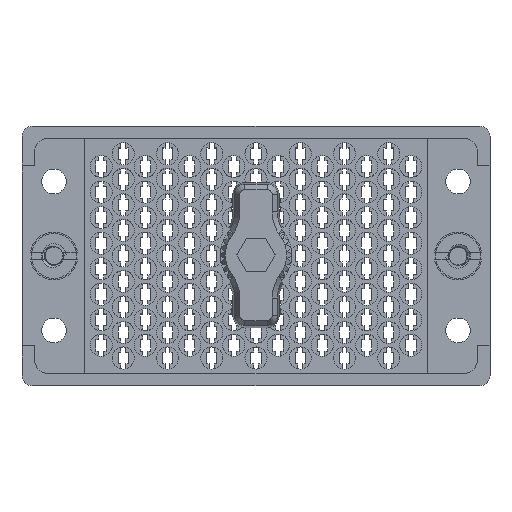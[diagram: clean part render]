
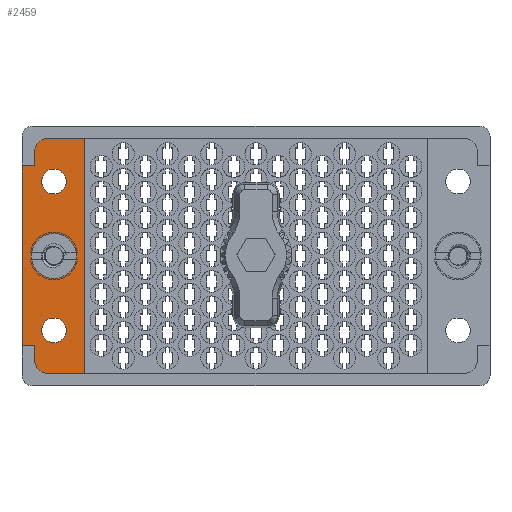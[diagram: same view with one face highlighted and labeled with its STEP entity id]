
A CAD part, top view. The second image highlights one B-rep face of the part: STEP entity #2459.
In plain terms, the highlighted planar face has unit normal (0, 0, 1).
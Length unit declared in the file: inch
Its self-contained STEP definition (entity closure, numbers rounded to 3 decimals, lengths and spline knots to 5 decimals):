
#202 = DIRECTION ( 'NONE',  ( 0., 0., 1. ) ) ;
#1156 = AXIS2_PLACEMENT_3D ( 'NONE', #48241, #108371, #100209 ) ;
#2459 = ADVANCED_FACE ( 'NONE', ( #61265, #38686, #32164, #97308 ), #48688, .T. ) ;
#4063 = DIRECTION ( 'NONE',  ( 0., 0., 1. ) ) ;
#4289 = EDGE_CURVE ( 'NONE', #85625, #64755, #30792, .T. ) ;
#6170 = ORIENTED_EDGE ( 'NONE', *, *, #50398, .F. ) ;
#6669 = CARTESIAN_POINT ( 'NONE',  ( -1.26, 0.4375, -0.117 ) ) ;
#8093 = CIRCLE ( 'NONE', #88939, 0.075 ) ;
#9647 = EDGE_LOOP ( 'NONE', ( #76361, #94280 ) ) ;
#10760 = ORIENTED_EDGE ( 'NONE', *, *, #34440, .T. ) ;
#11566 = LINE ( 'NONE', #105293, #71354 ) ;
#12044 = ORIENTED_EDGE ( 'NONE', *, *, #94939, .T. ) ;
#12897 = CARTESIAN_POINT ( 'NONE',  ( -1.3, 0., -0.117 ) ) ;
#13756 = CARTESIAN_POINT ( 'NONE',  ( -1.225, 0.69, -0.117 ) ) ;
#14881 = DIRECTION ( 'NONE',  ( 1., 0., 0. ) ) ;
#16908 = LINE ( 'NONE', #58837, #104635 ) ;
#18462 = LINE ( 'NONE', #58819, #83582 ) ;
#19349 = DIRECTION ( 'NONE',  ( 0., 0., 1. ) ) ;
#20358 = AXIS2_PLACEMENT_3D ( 'NONE', #100452, #58110, #75189 ) ;
#21151 = DIRECTION ( 'NONE',  ( 1., 0., 0. ) ) ;
#21687 = DIRECTION ( 'NONE',  ( 1., 0., 0. ) ) ;
#23961 = EDGE_LOOP ( 'NONE', ( #100579, #12044, #10760, #46238, #97655, #6170, #43141, #68533, #96807, #47739 ) ) ;
#24908 = CARTESIAN_POINT ( 'NONE',  ( -1.32, 0., -0.117 ) ) ;
#25008 = VERTEX_POINT ( 'NONE', #60267 ) ;
#25371 = VERTEX_POINT ( 'NONE', #107013 ) ;
#26425 = EDGE_LOOP ( 'NONE', ( #42098, #32777 ) ) ;
#26443 = LINE ( 'NONE', #81622, #51700 ) ;
#27898 = CARTESIAN_POINT ( 'NONE',  ( -1.1875, -0.4375, -0.117 ) ) ;
#30718 = EDGE_CURVE ( 'NONE', #97364, #71471, #67010, .T. ) ;
#30792 = LINE ( 'NONE', #44083, #95869 ) ;
#30960 = CARTESIAN_POINT ( 'NONE',  ( -1.005, 0.69, -0.117 ) ) ;
#32164 = FACE_BOUND ( 'NONE', #9647, .T. ) ;
#32777 = ORIENTED_EDGE ( 'NONE', *, *, #61422, .F. ) ;
#33132 = EDGE_CURVE ( 'NONE', #85235, #85625, #18462, .T. ) ;
#33253 = CIRCLE ( 'NONE', #103457, 0.0725 ) ;
#33356 = VECTOR ( 'NONE', #58072, 39.37008 ) ;
#33606 = VERTEX_POINT ( 'NONE', #6669 ) ;
#33649 = VERTEX_POINT ( 'NONE', #67560 ) ;
#33679 = LINE ( 'NONE', #75118, #60197 ) ;
#34440 = EDGE_CURVE ( 'NONE', #106465, #25008, #11566, .T. ) ;
#34630 = LINE ( 'NONE', #100408, #33356 ) ;
#36537 = AXIS2_PLACEMENT_3D ( 'NONE', #27898, #19349, #95850 ) ;
#37973 = DIRECTION ( 'NONE',  ( 1., 0., 0. ) ) ;
#38686 = FACE_BOUND ( 'NONE', #26425, .T. ) ;
#42098 = ORIENTED_EDGE ( 'NONE', *, *, #30718, .F. ) ;
#43141 = ORIENTED_EDGE ( 'NONE', *, *, #59621, .T. ) ;
#44083 = CARTESIAN_POINT ( 'NONE',  ( 0., 0.69, -0.117 ) ) ;
#44820 = DIRECTION ( 'NONE',  ( -1., 0., 0. ) ) ;
#46238 = ORIENTED_EDGE ( 'NONE', *, *, #93476, .T. ) ;
#47739 = ORIENTED_EDGE ( 'NONE', *, *, #33132, .T. ) ;
#47819 = EDGE_LOOP ( 'NONE', ( #90744, #95630 ) ) ;
#48241 = CARTESIAN_POINT ( 'NONE',  ( -1.225, 0.615, -0.117 ) ) ;
#48542 = AXIS2_PLACEMENT_3D ( 'NONE', #62396, #4063, #21151 ) ;
#48688 = PLANE ( 'NONE',  #60248 ) ;
#49027 = EDGE_CURVE ( 'NONE', #33649, #51265, #33679, .T. ) ;
#50398 = EDGE_CURVE ( 'NONE', #25371, #51265, #34630, .T. ) ;
#50629 = DIRECTION ( 'NONE',  ( 0., 1., 0. ) ) ;
#50853 = EDGE_CURVE ( 'NONE', #98989, #72801, #85011, .T. ) ;
#51251 = CARTESIAN_POINT ( 'NONE',  ( -1.3, -0.615, -0.117 ) ) ;
#51265 = VERTEX_POINT ( 'NONE', #78604 ) ;
#51700 = VECTOR ( 'NONE', #73082, 39.37008 ) ;
#53683 = DIRECTION ( 'NONE',  ( 0., -1., 0. ) ) ;
#55628 = DIRECTION ( 'NONE',  ( 0., -1., 0. ) ) ;
#56229 = DIRECTION ( 'NONE',  ( 0., 0., 1. ) ) ;
#58072 = DIRECTION ( 'NONE',  ( -1., 0., 0. ) ) ;
#58110 = DIRECTION ( 'NONE',  ( 0., 0., 1. ) ) ;
#58331 = DIRECTION ( 'NONE',  ( 0., 0., 1. ) ) ;
#58819 = CARTESIAN_POINT ( 'NONE',  ( -1.005, 0.7625, -0.117 ) ) ;
#58837 = CARTESIAN_POINT ( 'NONE',  ( 0., -0.69, -0.117 ) ) ;
#59216 = AXIS2_PLACEMENT_3D ( 'NONE', #93768, #202, #68166 ) ;
#59621 = EDGE_CURVE ( 'NONE', #25371, #102168, #61151, .T. ) ;
#60197 = VECTOR ( 'NONE', #74015, 39.37008 ) ;
#60248 = AXIS2_PLACEMENT_3D ( 'NONE', #108091, #58331, #14881 ) ;
#60267 = CARTESIAN_POINT ( 'NONE',  ( -1.3, 0.5285, -0.117 ) ) ;
#61151 = LINE ( 'NONE', #12897, #66470 ) ;
#61265 = FACE_BOUND ( 'NONE', #47819, .T. ) ;
#61422 = EDGE_CURVE ( 'NONE', #71471, #97364, #64324, .T. ) ;
#62396 = CARTESIAN_POINT ( 'NONE',  ( -1.1875, 0., -0.117 ) ) ;
#64324 = CIRCLE ( 'NONE', #36537, 0.0725 ) ;
#64660 = DIRECTION ( 'NONE',  ( 0., 0., 1. ) ) ;
#64667 = VERTEX_POINT ( 'NONE', #79921 ) ;
#64755 = VERTEX_POINT ( 'NONE', #13756 ) ;
#65998 = CIRCLE ( 'NONE', #1156, 0.075 ) ;
#66470 = VECTOR ( 'NONE', #55628, 39.37008 ) ;
#66790 = DIRECTION ( 'NONE',  ( 1., 0., 0. ) ) ;
#67010 = CIRCLE ( 'NONE', #59216, 0.0725 ) ;
#67349 = DIRECTION ( 'NONE',  ( -1., 0., 0. ) ) ;
#67560 = CARTESIAN_POINT ( 'NONE',  ( -1.375, 0.5285, -0.117 ) ) ;
#68004 = CARTESIAN_POINT ( 'NONE',  ( -1.115, -0.4375, -0.117 ) ) ;
#68166 = DIRECTION ( 'NONE',  ( 1., 0., 0. ) ) ;
#68533 = ORIENTED_EDGE ( 'NONE', *, *, #75363, .T. ) ;
#69321 = CIRCLE ( 'NONE', #20358, 0.1325 ) ;
#69415 = CARTESIAN_POINT ( 'NONE',  ( -1.26, -0.4375, -0.117 ) ) ;
#71354 = VECTOR ( 'NONE', #53683, 39.37008 ) ;
#71471 = VERTEX_POINT ( 'NONE', #68004 ) ;
#72801 = VERTEX_POINT ( 'NONE', #79033 ) ;
#73082 = DIRECTION ( 'NONE',  ( -1., 0., 0. ) ) ;
#73471 = EDGE_CURVE ( 'NONE', #33606, #64667, #93384, .T. ) ;
#74015 = DIRECTION ( 'NONE',  ( 0., -1., 0. ) ) ;
#75118 = CARTESIAN_POINT ( 'NONE',  ( -1.375, 0.7625, -0.117 ) ) ;
#75189 = DIRECTION ( 'NONE',  ( 1., 0., 0. ) ) ;
#75363 = EDGE_CURVE ( 'NONE', #102168, #97219, #8093, .T. ) ;
#76361 = ORIENTED_EDGE ( 'NONE', *, *, #104033, .F. ) ;
#77356 = CARTESIAN_POINT ( 'NONE',  ( -1.3, 0.615, -0.117 ) ) ;
#78604 = CARTESIAN_POINT ( 'NONE',  ( -1.375, -0.5285, -0.117 ) ) ;
#79033 = CARTESIAN_POINT ( 'NONE',  ( -1.055, 0., -0.117 ) ) ;
#79921 = CARTESIAN_POINT ( 'NONE',  ( -1.115, 0.4375, -0.117 ) ) ;
#81622 = CARTESIAN_POINT ( 'NONE',  ( 0., 0.5285, -0.117 ) ) ;
#83582 = VECTOR ( 'NONE', #50629, 39.37008 ) ;
#85011 = CIRCLE ( 'NONE', #48542, 0.1325 ) ;
#85235 = VERTEX_POINT ( 'NONE', #93771 ) ;
#85625 = VERTEX_POINT ( 'NONE', #30960 ) ;
#88939 = AXIS2_PLACEMENT_3D ( 'NONE', #92739, #109125, #66790 ) ;
#90744 = ORIENTED_EDGE ( 'NONE', *, *, #73471, .F. ) ;
#92422 = CARTESIAN_POINT ( 'NONE',  ( -1.225, -0.69, -0.117 ) ) ;
#92444 = AXIS2_PLACEMENT_3D ( 'NONE', #107095, #56229, #21687 ) ;
#92739 = CARTESIAN_POINT ( 'NONE',  ( -1.225, -0.615, -0.117 ) ) ;
#92798 = EDGE_CURVE ( 'NONE', #64667, #33606, #33253, .T. ) ;
#93384 = CIRCLE ( 'NONE', #92444, 0.0725 ) ;
#93476 = EDGE_CURVE ( 'NONE', #25008, #33649, #26443, .T. ) ;
#93768 = CARTESIAN_POINT ( 'NONE',  ( -1.1875, -0.4375, -0.117 ) ) ;
#93771 = CARTESIAN_POINT ( 'NONE',  ( -1.005, -0.69, -0.117 ) ) ;
#94280 = ORIENTED_EDGE ( 'NONE', *, *, #50853, .F. ) ;
#94939 = EDGE_CURVE ( 'NONE', #64755, #106465, #65998, .T. ) ;
#95630 = ORIENTED_EDGE ( 'NONE', *, *, #92798, .F. ) ;
#95850 = DIRECTION ( 'NONE',  ( 1., 0., 0. ) ) ;
#95869 = VECTOR ( 'NONE', #44820, 39.37008 ) ;
#96807 = ORIENTED_EDGE ( 'NONE', *, *, #109407, .F. ) ;
#97219 = VERTEX_POINT ( 'NONE', #92422 ) ;
#97308 = FACE_OUTER_BOUND ( 'NONE', #23961, .T. ) ;
#97364 = VERTEX_POINT ( 'NONE', #69415 ) ;
#97655 = ORIENTED_EDGE ( 'NONE', *, *, #49027, .T. ) ;
#98989 = VERTEX_POINT ( 'NONE', #24908 ) ;
#100209 = DIRECTION ( 'NONE',  ( 1., 0., 0. ) ) ;
#100408 = CARTESIAN_POINT ( 'NONE',  ( 0., -0.5285, -0.117 ) ) ;
#100452 = CARTESIAN_POINT ( 'NONE',  ( -1.1875, 0., -0.117 ) ) ;
#100579 = ORIENTED_EDGE ( 'NONE', *, *, #4289, .T. ) ;
#102168 = VERTEX_POINT ( 'NONE', #51251 ) ;
#103457 = AXIS2_PLACEMENT_3D ( 'NONE', #106288, #64660, #37973 ) ;
#104033 = EDGE_CURVE ( 'NONE', #72801, #98989, #69321, .T. ) ;
#104635 = VECTOR ( 'NONE', #67349, 39.37008 ) ;
#105293 = CARTESIAN_POINT ( 'NONE',  ( -1.3, 0., -0.117 ) ) ;
#106288 = CARTESIAN_POINT ( 'NONE',  ( -1.1875, 0.4375, -0.117 ) ) ;
#106465 = VERTEX_POINT ( 'NONE', #77356 ) ;
#107013 = CARTESIAN_POINT ( 'NONE',  ( -1.3, -0.5285, -0.117 ) ) ;
#107095 = CARTESIAN_POINT ( 'NONE',  ( -1.1875, 0.4375, -0.117 ) ) ;
#108091 = CARTESIAN_POINT ( 'NONE',  ( -1.375, -0.7625, -0.117 ) ) ;
#108371 = DIRECTION ( 'NONE',  ( 0., 0., 1. ) ) ;
#109125 = DIRECTION ( 'NONE',  ( 0., 0., 1. ) ) ;
#109407 = EDGE_CURVE ( 'NONE', #85235, #97219, #16908, .T. ) ;
